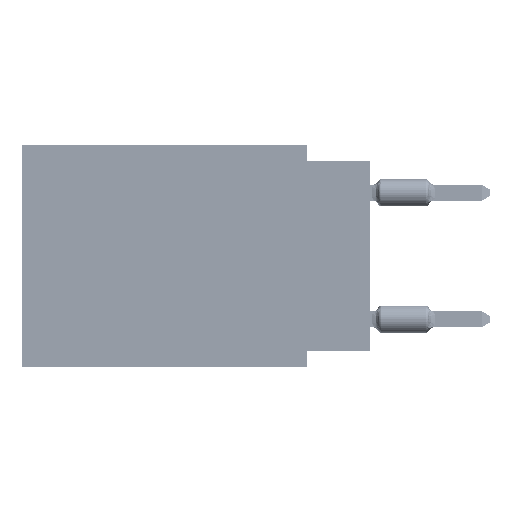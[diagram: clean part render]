
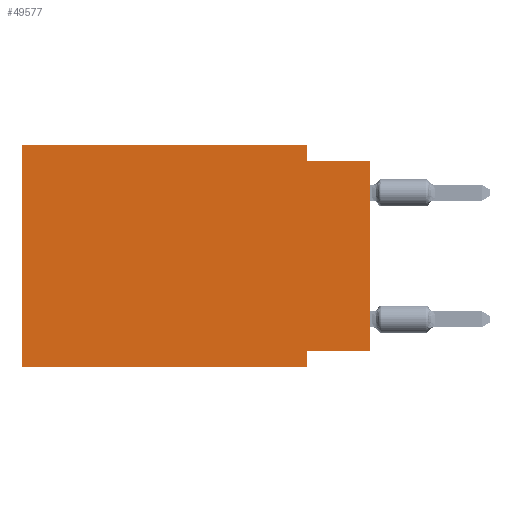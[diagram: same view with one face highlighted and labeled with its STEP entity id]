
A CAD part, left-side view. The second image highlights one B-rep face of the part: STEP entity #49577.
In plain terms, the highlighted planar face has unit normal (-1, 0, 0).
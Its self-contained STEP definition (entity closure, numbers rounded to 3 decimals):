
#2100 = ORIENTED_EDGE ( 'NONE', *, *, #40636, .F. ) ;
#2254 = LINE ( 'NONE', #53044, #10077 ) ;
#3805 = AXIS2_PLACEMENT_3D ( 'NONE', #19054, #33391, #54423 ) ;
#6457 = LINE ( 'NONE', #57219, #24019 ) ;
#8646 = CARTESIAN_POINT ( 'NONE',  ( 0., 0., 0. ) ) ;
#9634 = CARTESIAN_POINT ( 'NONE',  ( 0., 13.97, -8.89 ) ) ;
#10077 = VECTOR ( 'NONE', #48032, 1000. ) ;
#12264 = VECTOR ( 'NONE', #44844, 1000. ) ;
#14847 = ORIENTED_EDGE ( 'NONE', *, *, #40447, .F. ) ;
#16263 = LINE ( 'NONE', #56989, #21192 ) ;
#17144 = DIRECTION ( 'NONE',  ( 0., 0., -1. ) ) ;
#17202 = VECTOR ( 'NONE', #34059, 1000. ) ;
#18691 = LINE ( 'NONE', #8646, #17202 ) ;
#19054 = CARTESIAN_POINT ( 'NONE',  ( 0., 13.97, 0. ) ) ;
#20084 = CARTESIAN_POINT ( 'NONE',  ( 0., 2.54, -0.635 ) ) ;
#21192 = VECTOR ( 'NONE', #25632, 1000. ) ;
#21737 = CARTESIAN_POINT ( 'NONE',  ( 0., 0., -8.255 ) ) ;
#22039 = ORIENTED_EDGE ( 'NONE', *, *, #42572, .F. ) ;
#22055 = VECTOR ( 'NONE', #28189, 1000. ) ;
#23868 = ORIENTED_EDGE ( 'NONE', *, *, #65189, .T. ) ;
#24019 = VECTOR ( 'NONE', #17144, 1000. ) ;
#25632 = DIRECTION ( 'NONE',  ( 0., 0., 1. ) ) ;
#27507 = VERTEX_POINT ( 'NONE', #28501 ) ;
#28189 = DIRECTION ( 'NONE',  ( 0., 1., 0. ) ) ;
#28501 = CARTESIAN_POINT ( 'NONE',  ( 0., 2.54, -8.255 ) ) ;
#28731 = FACE_OUTER_BOUND ( 'NONE', #40436, .T. ) ;
#30012 = DIRECTION ( 'NONE',  ( 0., -1., 0. ) ) ;
#30092 = DIRECTION ( 'NONE',  ( 0., 0., -1. ) ) ;
#30177 = ORIENTED_EDGE ( 'NONE', *, *, #55771, .F. ) ;
#31632 = CARTESIAN_POINT ( 'NONE',  ( 0., 0., -0.635 ) ) ;
#33166 = LINE ( 'NONE', #53526, #12264 ) ;
#33391 = DIRECTION ( 'NONE',  ( 1., 0., 0. ) ) ;
#34059 = DIRECTION ( 'NONE',  ( 0., 0., 1. ) ) ;
#35391 = EDGE_CURVE ( 'NONE', #55125, #54060, #2254, .T. ) ;
#37046 = CARTESIAN_POINT ( 'NONE',  ( 0., 13.97, 0. ) ) ;
#38003 = CARTESIAN_POINT ( 'NONE',  ( 0., 2.54, 0. ) ) ;
#38518 = VECTOR ( 'NONE', #30012, 1000. ) ;
#38781 = ORIENTED_EDGE ( 'NONE', *, *, #65222, .T. ) ;
#40134 = CARTESIAN_POINT ( 'NONE',  ( 0., 2.54, -8.89 ) ) ;
#40436 = EDGE_LOOP ( 'NONE', ( #38781, #46202, #14847, #2100, #61712, #23868, #22039, #30177 ) ) ;
#40447 = EDGE_CURVE ( 'NONE', #63415, #55125, #6457, .T. ) ;
#40470 = LINE ( 'NONE', #40134, #47664 ) ;
#40636 = EDGE_CURVE ( 'NONE', #41161, #63415, #33166, .T. ) ;
#41161 = VERTEX_POINT ( 'NONE', #37046 ) ;
#42572 = EDGE_CURVE ( 'NONE', #27507, #45123, #40470, .T. ) ;
#43234 = LINE ( 'NONE', #63599, #22055 ) ;
#44641 = CARTESIAN_POINT ( 'NONE',  ( 0., 13.97, -8.89 ) ) ;
#44844 = DIRECTION ( 'NONE',  ( 0., -1., 0. ) ) ;
#45123 = VERTEX_POINT ( 'NONE', #50908 ) ;
#46202 = ORIENTED_EDGE ( 'NONE', *, *, #35391, .F. ) ;
#47664 = VECTOR ( 'NONE', #30092, 1000. ) ;
#48032 = DIRECTION ( 'NONE',  ( 0., -1., 0. ) ) ;
#49099 = PLANE ( 'NONE',  #3805 ) ;
#49400 = VERTEX_POINT ( 'NONE', #21737 ) ;
#49577 = ADVANCED_FACE ( 'NONE', ( #28731 ), #49099, .F. ) ;
#50908 = CARTESIAN_POINT ( 'NONE',  ( 0., 2.54, -8.89 ) ) ;
#53044 = CARTESIAN_POINT ( 'NONE',  ( 0., 0., -0.635 ) ) ;
#53526 = CARTESIAN_POINT ( 'NONE',  ( 0., 13.97, 0. ) ) ;
#54060 = VERTEX_POINT ( 'NONE', #31632 ) ;
#54423 = DIRECTION ( 'NONE',  ( 0., 0., -1. ) ) ;
#55125 = VERTEX_POINT ( 'NONE', #20084 ) ;
#55771 = EDGE_CURVE ( 'NONE', #49400, #27507, #43234, .T. ) ;
#56989 = CARTESIAN_POINT ( 'NONE',  ( 0., 13.97, 0. ) ) ;
#57219 = CARTESIAN_POINT ( 'NONE',  ( 0., 2.54, 0. ) ) ;
#59434 = LINE ( 'NONE', #9634, #38518 ) ;
#60089 = EDGE_CURVE ( 'NONE', #61615, #41161, #16263, .T. ) ;
#61615 = VERTEX_POINT ( 'NONE', #44641 ) ;
#61712 = ORIENTED_EDGE ( 'NONE', *, *, #60089, .F. ) ;
#63415 = VERTEX_POINT ( 'NONE', #38003 ) ;
#63599 = CARTESIAN_POINT ( 'NONE',  ( 0., 0., -8.255 ) ) ;
#65189 = EDGE_CURVE ( 'NONE', #61615, #45123, #59434, .T. ) ;
#65222 = EDGE_CURVE ( 'NONE', #49400, #54060, #18691, .T. ) ;
